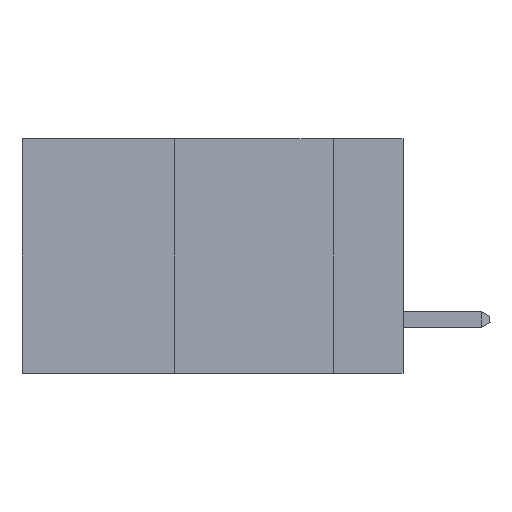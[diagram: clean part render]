
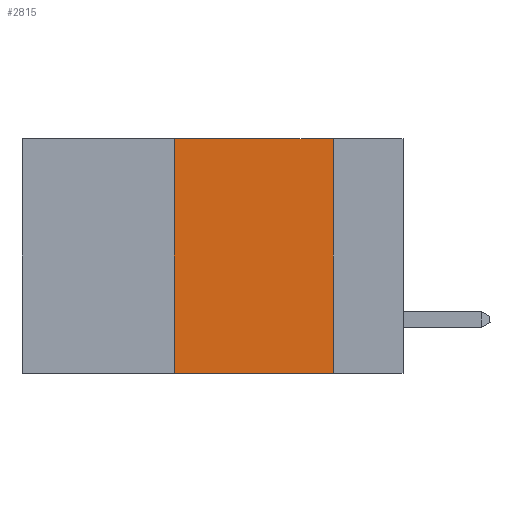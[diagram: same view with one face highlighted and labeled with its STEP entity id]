
A CAD part, left-side view. The second image highlights one B-rep face of the part: STEP entity #2815.
In plain terms, the highlighted planar face has unit normal (-1, 0, 0).
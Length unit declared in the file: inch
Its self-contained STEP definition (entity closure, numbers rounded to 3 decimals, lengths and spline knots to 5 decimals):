
#670 = CARTESIAN_POINT ( 'NONE',  ( 0., 0.36, -0.37 ) ) ;
#2815 = ADVANCED_FACE ( 'NONE', ( #45662 ), #6498, .F. ) ;
#2832 = CARTESIAN_POINT ( 'NONE',  ( 0., 0.6, 0. ) ) ;
#3135 = EDGE_CURVE ( 'NONE', #14586, #45979, #22542, .T. ) ;
#3313 = CARTESIAN_POINT ( 'NONE',  ( 0., 0.36, 0. ) ) ;
#6498 = PLANE ( 'NONE',  #36543 ) ;
#7089 = CARTESIAN_POINT ( 'NONE',  ( 0., 0.6, 0. ) ) ;
#7409 = DIRECTION ( 'NONE',  ( 0., -1., 0. ) ) ;
#11646 = EDGE_LOOP ( 'NONE', ( #42891, #26717, #13843, #46048 ) ) ;
#13843 = ORIENTED_EDGE ( 'NONE', *, *, #32647, .F. ) ;
#13998 = CARTESIAN_POINT ( 'NONE',  ( 0., 0.36, 0. ) ) ;
#14272 = LINE ( 'NONE', #14382, #14859 ) ;
#14382 = CARTESIAN_POINT ( 'NONE',  ( 0., 0.6, -0.37 ) ) ;
#14412 = CARTESIAN_POINT ( 'NONE',  ( 0., 0.11, -0.37 ) ) ;
#14586 = VERTEX_POINT ( 'NONE', #13998 ) ;
#14859 = VECTOR ( 'NONE', #44156, 39.37008 ) ;
#21134 = DIRECTION ( 'NONE',  ( 0., 0., -1. ) ) ;
#21920 = VECTOR ( 'NONE', #21134, 39.37008 ) ;
#22402 = DIRECTION ( 'NONE',  ( 0., 0., 1. ) ) ;
#22542 = LINE ( 'NONE', #7089, #36088 ) ;
#22546 = VECTOR ( 'NONE', #22402, 39.37008 ) ;
#24886 = LINE ( 'NONE', #36313, #21920 ) ;
#25227 = DIRECTION ( 'NONE',  ( 0., 0., -1. ) ) ;
#26040 = CARTESIAN_POINT ( 'NONE',  ( 0., 0.11, 0. ) ) ;
#26717 = ORIENTED_EDGE ( 'NONE', *, *, #3135, .F. ) ;
#29371 = DIRECTION ( 'NONE',  ( 1., 0., 0. ) ) ;
#32647 = EDGE_CURVE ( 'NONE', #42849, #14586, #33206, .T. ) ;
#32673 = EDGE_CURVE ( 'NONE', #42849, #43933, #14272, .T. ) ;
#33206 = LINE ( 'NONE', #3313, #22546 ) ;
#36088 = VECTOR ( 'NONE', #7409, 39.37008 ) ;
#36313 = CARTESIAN_POINT ( 'NONE',  ( 0., 0.11, 0. ) ) ;
#36543 = AXIS2_PLACEMENT_3D ( 'NONE', #2832, #29371, #25227 ) ;
#42849 = VERTEX_POINT ( 'NONE', #670 ) ;
#42891 = ORIENTED_EDGE ( 'NONE', *, *, #44420, .F. ) ;
#43933 = VERTEX_POINT ( 'NONE', #14412 ) ;
#44156 = DIRECTION ( 'NONE',  ( 0., -1., 0. ) ) ;
#44420 = EDGE_CURVE ( 'NONE', #45979, #43933, #24886, .T. ) ;
#45662 = FACE_OUTER_BOUND ( 'NONE', #11646, .T. ) ;
#45979 = VERTEX_POINT ( 'NONE', #26040 ) ;
#46048 = ORIENTED_EDGE ( 'NONE', *, *, #32673, .T. ) ;
